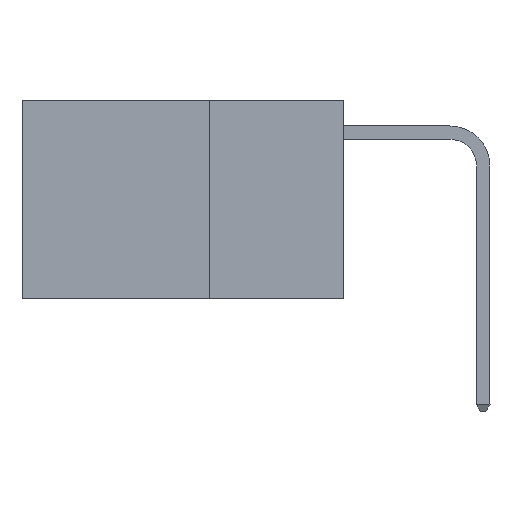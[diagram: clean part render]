
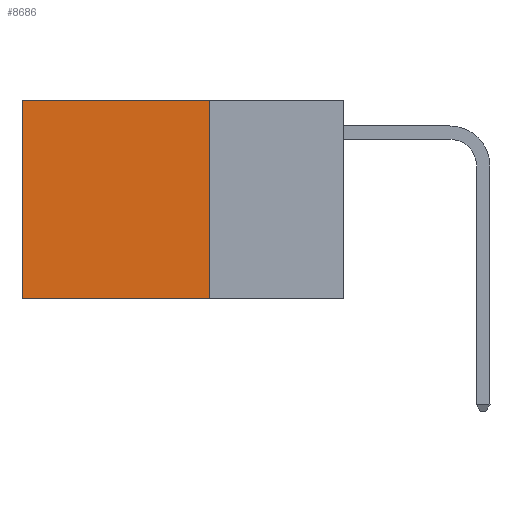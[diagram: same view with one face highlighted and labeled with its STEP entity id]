
A CAD part, left-side view. The second image highlights one B-rep face of the part: STEP entity #8686.
In plain terms, the highlighted planar face has unit normal (-1, 0, 0).
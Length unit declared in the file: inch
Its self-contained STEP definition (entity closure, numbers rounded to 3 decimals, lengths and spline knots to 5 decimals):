
#965 = CARTESIAN_POINT ( 'NONE',  ( 0.2625, 0.25, 0. ) ) ;
#1141 = CARTESIAN_POINT ( 'NONE',  ( 0.2625, 0.25, -0.37 ) ) ;
#1240 = LINE ( 'NONE', #1141, #16843 ) ;
#1753 = CARTESIAN_POINT ( 'NONE',  ( 0.2625, 0.25, 0. ) ) ;
#2346 = CARTESIAN_POINT ( 'NONE',  ( 0.2625, 0.6, 0. ) ) ;
#3850 = LINE ( 'NONE', #2346, #14899 ) ;
#4918 = ORIENTED_EDGE ( 'NONE', *, *, #19037, .F. ) ;
#5062 = DIRECTION ( 'NONE',  ( 0., 0., -1. ) ) ;
#5608 = EDGE_CURVE ( 'NONE', #11223, #7639, #10856, .T. ) ;
#6829 = ORIENTED_EDGE ( 'NONE', *, *, #5608, .T. ) ;
#6976 = EDGE_CURVE ( 'NONE', #7639, #9078, #3850, .T. ) ;
#7149 = DIRECTION ( 'NONE',  ( 1., 0., 0. ) ) ;
#7256 = FACE_OUTER_BOUND ( 'NONE', #17762, .T. ) ;
#7518 = CARTESIAN_POINT ( 'NONE',  ( 0.2625, 0.6, 0. ) ) ;
#7639 = VERTEX_POINT ( 'NONE', #7518 ) ;
#7807 = ORIENTED_EDGE ( 'NONE', *, *, #8567, .F. ) ;
#8442 = DIRECTION ( 'NONE',  ( 0., 0., -1. ) ) ;
#8567 = EDGE_CURVE ( 'NONE', #11223, #10979, #17363, .T. ) ;
#8686 = ADVANCED_FACE ( 'NONE', ( #7256 ), #14552, .F. ) ;
#9078 = VERTEX_POINT ( 'NONE', #9900 ) ;
#9900 = CARTESIAN_POINT ( 'NONE',  ( 0.2625, 0.6, -0.37 ) ) ;
#10416 = DIRECTION ( 'NONE',  ( 0., 1., 0. ) ) ;
#10754 = CARTESIAN_POINT ( 'NONE',  ( 0.2625, 0.25, 0. ) ) ;
#10856 = LINE ( 'NONE', #1753, #10998 ) ;
#10979 = VERTEX_POINT ( 'NONE', #16383 ) ;
#10998 = VECTOR ( 'NONE', #11142, 39.37008 ) ;
#11142 = DIRECTION ( 'NONE',  ( 0., 1., 0. ) ) ;
#11223 = VERTEX_POINT ( 'NONE', #10754 ) ;
#13327 = VECTOR ( 'NONE', #5062, 39.37008 ) ;
#14252 = CARTESIAN_POINT ( 'NONE',  ( 0.2625, 0.25, 0. ) ) ;
#14552 = PLANE ( 'NONE',  #17503 ) ;
#14899 = VECTOR ( 'NONE', #8442, 39.37008 ) ;
#16383 = CARTESIAN_POINT ( 'NONE',  ( 0.2625, 0.25, -0.37 ) ) ;
#16740 = ORIENTED_EDGE ( 'NONE', *, *, #6976, .T. ) ;
#16843 = VECTOR ( 'NONE', #10416, 39.37008 ) ;
#17363 = LINE ( 'NONE', #14252, #13327 ) ;
#17503 = AXIS2_PLACEMENT_3D ( 'NONE', #965, #7149, #19474 ) ;
#17762 = EDGE_LOOP ( 'NONE', ( #16740, #4918, #7807, #6829 ) ) ;
#19037 = EDGE_CURVE ( 'NONE', #10979, #9078, #1240, .T. ) ;
#19474 = DIRECTION ( 'NONE',  ( 0., 0., -1. ) ) ;
